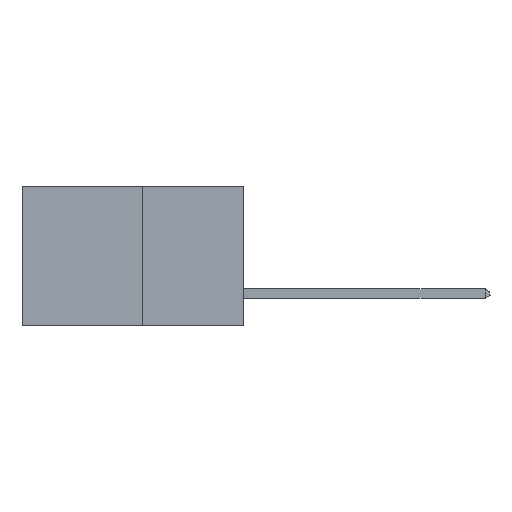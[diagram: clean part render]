
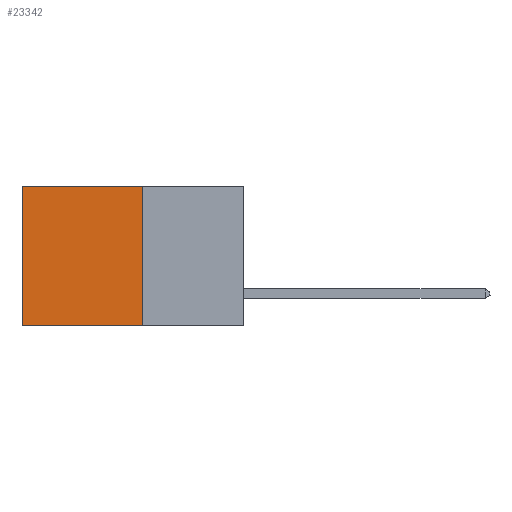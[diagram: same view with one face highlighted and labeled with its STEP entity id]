
A CAD part, left-side view. The second image highlights one B-rep face of the part: STEP entity #23342.
In plain terms, the highlighted planar face has unit normal (-1, 0, 0).
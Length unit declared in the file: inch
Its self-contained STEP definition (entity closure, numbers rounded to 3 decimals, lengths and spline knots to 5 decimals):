
#1932 = CARTESIAN_POINT ( 'NONE',  ( 0.277, 0.59, -0.37 ) ) ;
#3225 = EDGE_CURVE ( 'NONE', #22748, #10116, #19420, .T. ) ;
#3306 = EDGE_CURVE ( 'NONE', #3432, #10116, #17341, .T. ) ;
#3432 = VERTEX_POINT ( 'NONE', #20026 ) ;
#4035 = CARTESIAN_POINT ( 'NONE',  ( 0.277, 0.27, -0.37 ) ) ;
#4170 = CARTESIAN_POINT ( 'NONE',  ( 0.277, 0.27, -0.37 ) ) ;
#4657 = AXIS2_PLACEMENT_3D ( 'NONE', #4035, #19603, #6287 ) ;
#5321 = VECTOR ( 'NONE', #25286, 39.37008 ) ;
#6287 = DIRECTION ( 'NONE',  ( 0., 0., -1. ) ) ;
#7230 = ORIENTED_EDGE ( 'NONE', *, *, #16274, .F. ) ;
#7717 = ORIENTED_EDGE ( 'NONE', *, *, #3306, .T. ) ;
#8565 = DIRECTION ( 'NONE',  ( 0., 0., -1. ) ) ;
#10116 = VERTEX_POINT ( 'NONE', #22645 ) ;
#11506 = VERTEX_POINT ( 'NONE', #24993 ) ;
#11598 = ORIENTED_EDGE ( 'NONE', *, *, #27817, .T. ) ;
#11982 = DIRECTION ( 'NONE',  ( 0., 0., -1. ) ) ;
#14212 = VECTOR ( 'NONE', #15074, 39.37008 ) ;
#14639 = EDGE_LOOP ( 'NONE', ( #7717, #21651, #7230, #11598 ) ) ;
#15074 = DIRECTION ( 'NONE',  ( 0., 1., 0. ) ) ;
#15141 = PLANE ( 'NONE',  #4657 ) ;
#16274 = EDGE_CURVE ( 'NONE', #11506, #22748, #16395, .T. ) ;
#16395 = LINE ( 'NONE', #20806, #21578 ) ;
#17341 = LINE ( 'NONE', #1932, #23259 ) ;
#19420 = LINE ( 'NONE', #28275, #14212 ) ;
#19603 = DIRECTION ( 'NONE',  ( 1., 0., 0. ) ) ;
#20026 = CARTESIAN_POINT ( 'NONE',  ( 0.277, 0.59, 0. ) ) ;
#20806 = CARTESIAN_POINT ( 'NONE',  ( 0.277, 0.27, -0.37 ) ) ;
#21578 = VECTOR ( 'NONE', #11982, 39.37008 ) ;
#21651 = ORIENTED_EDGE ( 'NONE', *, *, #3225, .F. ) ;
#22645 = CARTESIAN_POINT ( 'NONE',  ( 0.277, 0.59, -0.37 ) ) ;
#22690 = FACE_OUTER_BOUND ( 'NONE', #14639, .T. ) ;
#22748 = VERTEX_POINT ( 'NONE', #4170 ) ;
#23057 = LINE ( 'NONE', #23076, #5321 ) ;
#23076 = CARTESIAN_POINT ( 'NONE',  ( 0.277, 0.27, 0. ) ) ;
#23259 = VECTOR ( 'NONE', #8565, 39.37008 ) ;
#23342 = ADVANCED_FACE ( 'NONE', ( #22690 ), #15141, .F. ) ;
#24993 = CARTESIAN_POINT ( 'NONE',  ( 0.277, 0.27, 0. ) ) ;
#25286 = DIRECTION ( 'NONE',  ( 0., 1., 0. ) ) ;
#27817 = EDGE_CURVE ( 'NONE', #11506, #3432, #23057, .T. ) ;
#28275 = CARTESIAN_POINT ( 'NONE',  ( 0.277, 0.27, -0.37 ) ) ;
